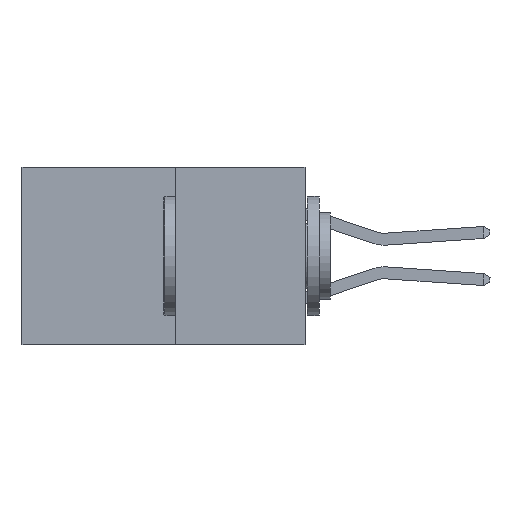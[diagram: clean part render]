
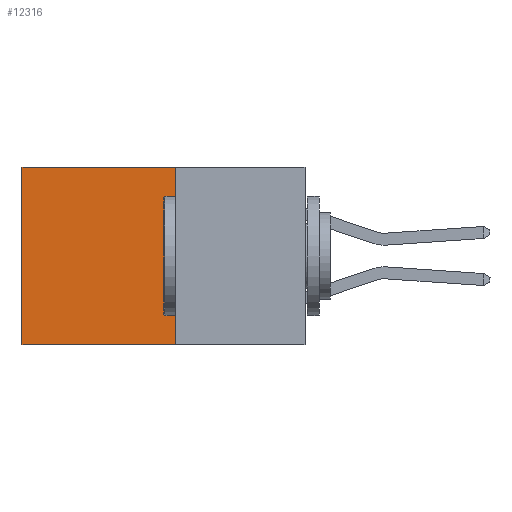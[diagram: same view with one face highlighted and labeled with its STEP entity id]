
A CAD part, left-side view. The second image highlights one B-rep face of the part: STEP entity #12316.
In plain terms, the highlighted planar face has unit normal (-1, 0, 0).
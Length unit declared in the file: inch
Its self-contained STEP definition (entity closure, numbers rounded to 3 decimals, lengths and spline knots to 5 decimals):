
#167 = VERTEX_POINT ( 'NONE', #6363 ) ;
#257 = CARTESIAN_POINT ( 'NONE',  ( 0.277, 0.27, 0. ) ) ;
#502 = CARTESIAN_POINT ( 'NONE',  ( 0.277, 0.27, -0.37 ) ) ;
#579 = ORIENTED_EDGE ( 'NONE', *, *, #18619, .T. ) ;
#1375 = VECTOR ( 'NONE', #2470, 39.37008 ) ;
#2042 = CARTESIAN_POINT ( 'NONE',  ( 0.277, 0.59, -0.37 ) ) ;
#2470 = DIRECTION ( 'NONE',  ( 0., 0., -1. ) ) ;
#3209 = LINE ( 'NONE', #18748, #22620 ) ;
#4360 = LINE ( 'NONE', #10585, #24325 ) ;
#4625 = EDGE_CURVE ( 'NONE', #167, #11171, #3209, .T. ) ;
#5503 = DIRECTION ( 'NONE',  ( 1., 0., 0. ) ) ;
#5555 = FACE_OUTER_BOUND ( 'NONE', #9023, .T. ) ;
#6363 = CARTESIAN_POINT ( 'NONE',  ( 0.277, 0.27, -0.37 ) ) ;
#7015 = ORIENTED_EDGE ( 'NONE', *, *, #19717, .T. ) ;
#7368 = CARTESIAN_POINT ( 'NONE',  ( 0.277, 0.59, 0. ) ) ;
#8272 = AXIS2_PLACEMENT_3D ( 'NONE', #15183, #5503, #19087 ) ;
#9023 = EDGE_LOOP ( 'NONE', ( #579, #10955, #11575, #7015 ) ) ;
#10585 = CARTESIAN_POINT ( 'NONE',  ( 0.277, 0.27, 0. ) ) ;
#10955 = ORIENTED_EDGE ( 'NONE', *, *, #4625, .F. ) ;
#11096 = VECTOR ( 'NONE', #15117, 39.37008 ) ;
#11171 = VERTEX_POINT ( 'NONE', #2042 ) ;
#11575 = ORIENTED_EDGE ( 'NONE', *, *, #17696, .F. ) ;
#12316 = ADVANCED_FACE ( 'NONE', ( #5555 ), #13245, .F. ) ;
#13179 = CARTESIAN_POINT ( 'NONE',  ( 0.277, 0.59, -0.37 ) ) ;
#13245 = PLANE ( 'NONE',  #8272 ) ;
#13871 = VERTEX_POINT ( 'NONE', #257 ) ;
#15117 = DIRECTION ( 'NONE',  ( 0., 0., -1. ) ) ;
#15183 = CARTESIAN_POINT ( 'NONE',  ( 0.277, 0.27, -0.37 ) ) ;
#16443 = DIRECTION ( 'NONE',  ( 0., 1., 0. ) ) ;
#16915 = LINE ( 'NONE', #502, #1375 ) ;
#17696 = EDGE_CURVE ( 'NONE', #13871, #167, #16915, .T. ) ;
#18619 = EDGE_CURVE ( 'NONE', #19250, #11171, #21381, .T. ) ;
#18748 = CARTESIAN_POINT ( 'NONE',  ( 0.277, 0.27, -0.37 ) ) ;
#18984 = DIRECTION ( 'NONE',  ( 0., 1., 0. ) ) ;
#19087 = DIRECTION ( 'NONE',  ( 0., 0., -1. ) ) ;
#19250 = VERTEX_POINT ( 'NONE', #7368 ) ;
#19717 = EDGE_CURVE ( 'NONE', #13871, #19250, #4360, .T. ) ;
#21381 = LINE ( 'NONE', #13179, #11096 ) ;
#22620 = VECTOR ( 'NONE', #18984, 39.37008 ) ;
#24325 = VECTOR ( 'NONE', #16443, 39.37008 ) ;
